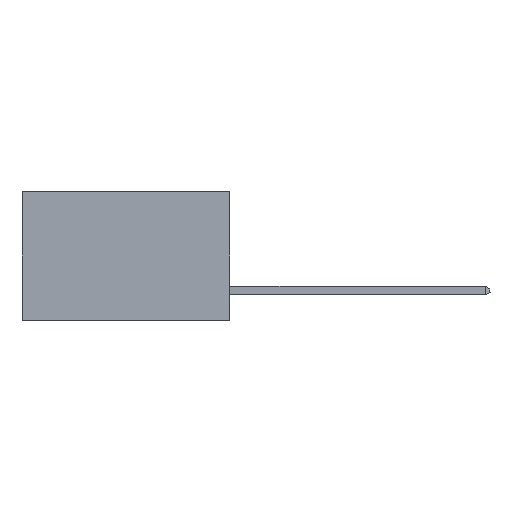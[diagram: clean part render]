
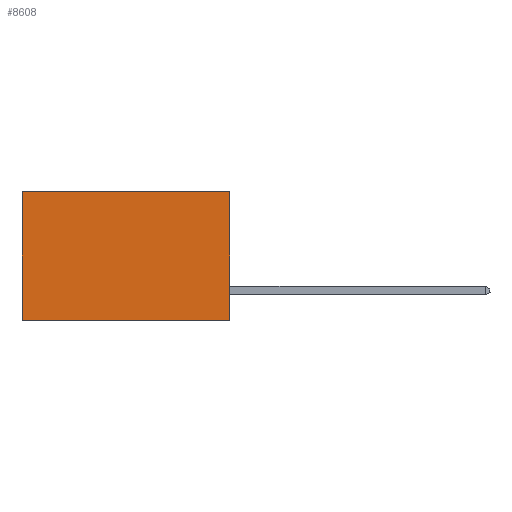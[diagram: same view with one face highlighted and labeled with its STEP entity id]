
A CAD part, left-side view. The second image highlights one B-rep face of the part: STEP entity #8608.
In plain terms, the highlighted planar face has unit normal (-1, 0, 0).
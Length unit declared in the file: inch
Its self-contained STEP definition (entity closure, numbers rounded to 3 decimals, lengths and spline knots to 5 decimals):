
#528 = LINE ( 'NONE', #7194, #631 ) ;
#631 = VECTOR ( 'NONE', #711, 39.37008 ) ;
#711 = DIRECTION ( 'NONE',  ( 0., 1., 0. ) ) ;
#1287 = FACE_OUTER_BOUND ( 'NONE', #2515, .T. ) ;
#1980 = DIRECTION ( 'NONE',  ( 0., 0., -1. ) ) ;
#2250 = VERTEX_POINT ( 'NONE', #6493 ) ;
#2435 = EDGE_CURVE ( 'NONE', #2975, #7603, #4480, .T. ) ;
#2515 = EDGE_LOOP ( 'NONE', ( #6610, #7405, #5896, #5111 ) ) ;
#2581 = CARTESIAN_POINT ( 'NONE',  ( 0.298, 0., -0.37 ) ) ;
#2638 = DIRECTION ( 'NONE',  ( 0., 1., 0. ) ) ;
#2810 = AXIS2_PLACEMENT_3D ( 'NONE', #4170, #7033, #9152 ) ;
#2975 = VERTEX_POINT ( 'NONE', #4937 ) ;
#3309 = EDGE_CURVE ( 'NONE', #2250, #7603, #4246, .T. ) ;
#3312 = CARTESIAN_POINT ( 'NONE',  ( 0.298, 0., 0. ) ) ;
#3804 = VERTEX_POINT ( 'NONE', #6172 ) ;
#4170 = CARTESIAN_POINT ( 'NONE',  ( 0.298, 0., 0. ) ) ;
#4246 = LINE ( 'NONE', #4956, #5638 ) ;
#4480 = LINE ( 'NONE', #2581, #6560 ) ;
#4676 = LINE ( 'NONE', #3312, #6987 ) ;
#4937 = CARTESIAN_POINT ( 'NONE',  ( 0.298, 0., -0.37 ) ) ;
#4956 = CARTESIAN_POINT ( 'NONE',  ( 0.298, 0.6, 0. ) ) ;
#5111 = ORIENTED_EDGE ( 'NONE', *, *, #8708, .T. ) ;
#5638 = VECTOR ( 'NONE', #1980, 39.37008 ) ;
#5896 = ORIENTED_EDGE ( 'NONE', *, *, #7891, .F. ) ;
#6172 = CARTESIAN_POINT ( 'NONE',  ( 0.298, 0., 0. ) ) ;
#6493 = CARTESIAN_POINT ( 'NONE',  ( 0.298, 0.6, 0. ) ) ;
#6560 = VECTOR ( 'NONE', #2638, 39.37008 ) ;
#6610 = ORIENTED_EDGE ( 'NONE', *, *, #3309, .T. ) ;
#6987 = VECTOR ( 'NONE', #7198, 39.37008 ) ;
#7003 = PLANE ( 'NONE',  #2810 ) ;
#7033 = DIRECTION ( 'NONE',  ( 1., 0., 0. ) ) ;
#7194 = CARTESIAN_POINT ( 'NONE',  ( 0.298, 0., 0. ) ) ;
#7198 = DIRECTION ( 'NONE',  ( 0., 0., -1. ) ) ;
#7351 = CARTESIAN_POINT ( 'NONE',  ( 0.298, 0.6, -0.37 ) ) ;
#7405 = ORIENTED_EDGE ( 'NONE', *, *, #2435, .F. ) ;
#7603 = VERTEX_POINT ( 'NONE', #7351 ) ;
#7891 = EDGE_CURVE ( 'NONE', #3804, #2975, #4676, .T. ) ;
#8608 = ADVANCED_FACE ( 'NONE', ( #1287 ), #7003, .F. ) ;
#8708 = EDGE_CURVE ( 'NONE', #3804, #2250, #528, .T. ) ;
#9152 = DIRECTION ( 'NONE',  ( 0., 0., -1. ) ) ;
